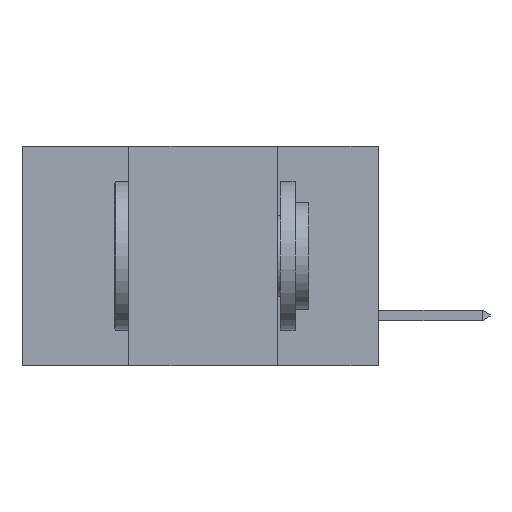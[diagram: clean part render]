
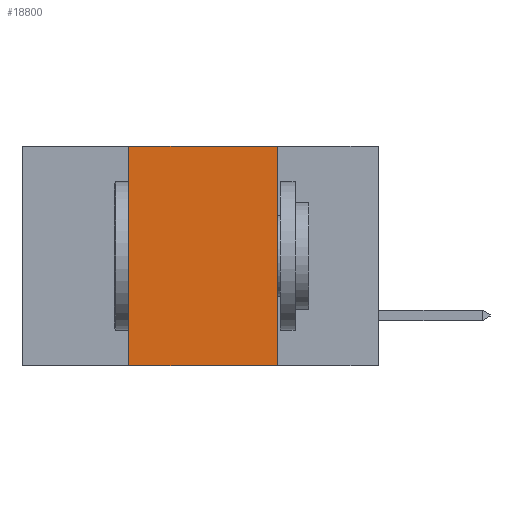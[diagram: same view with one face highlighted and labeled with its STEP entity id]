
A CAD part, left-side view. The second image highlights one B-rep face of the part: STEP entity #18800.
In plain terms, the highlighted planar face has unit normal (-1, 0, 0).
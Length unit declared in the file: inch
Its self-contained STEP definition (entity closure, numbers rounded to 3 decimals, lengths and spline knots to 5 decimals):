
#1243 = AXIS2_PLACEMENT_3D ( 'NONE', #8202, #19366, #8288 ) ;
#2293 = ORIENTED_EDGE ( 'NONE', *, *, #5641, .F. ) ;
#2319 = DIRECTION ( 'NONE',  ( 0., 0., 1. ) ) ;
#3098 = EDGE_CURVE ( 'NONE', #23307, #8638, #22812, .T. ) ;
#4354 = EDGE_CURVE ( 'NONE', #23307, #5265, #14156, .T. ) ;
#4547 = CARTESIAN_POINT ( 'NONE',  ( 0., 0.17, 0. ) ) ;
#5265 = VERTEX_POINT ( 'NONE', #8289 ) ;
#5309 = ORIENTED_EDGE ( 'NONE', *, *, #4354, .F. ) ;
#5473 = CARTESIAN_POINT ( 'NONE',  ( 0., 0.42, -0.37 ) ) ;
#5641 = EDGE_CURVE ( 'NONE', #20863, #8638, #9137, .T. ) ;
#6243 = FACE_OUTER_BOUND ( 'NONE', #12476, .T. ) ;
#6363 = PLANE ( 'NONE',  #1243 ) ;
#8202 = CARTESIAN_POINT ( 'NONE',  ( 0., 0.6, 0. ) ) ;
#8288 = DIRECTION ( 'NONE',  ( 0., 0., -1. ) ) ;
#8289 = CARTESIAN_POINT ( 'NONE',  ( 0., 0.42, 0. ) ) ;
#8351 = DIRECTION ( 'NONE',  ( 0., 0., -1. ) ) ;
#8638 = VERTEX_POINT ( 'NONE', #11165 ) ;
#9137 = LINE ( 'NONE', #4547, #23257 ) ;
#9141 = ORIENTED_EDGE ( 'NONE', *, *, #24098, .F. ) ;
#9716 = CARTESIAN_POINT ( 'NONE',  ( 0., 0.6, 0. ) ) ;
#11165 = CARTESIAN_POINT ( 'NONE',  ( 0., 0.17, -0.37 ) ) ;
#11465 = VECTOR ( 'NONE', #11610, 39.37008 ) ;
#11610 = DIRECTION ( 'NONE',  ( 0., -1., 0. ) ) ;
#11720 = CARTESIAN_POINT ( 'NONE',  ( 0., 0.6, -0.37 ) ) ;
#12476 = EDGE_LOOP ( 'NONE', ( #2293, #9141, #5309, #21863 ) ) ;
#12656 = CARTESIAN_POINT ( 'NONE',  ( 0., 0.17, 0. ) ) ;
#12867 = CARTESIAN_POINT ( 'NONE',  ( 0., 0.42, 0. ) ) ;
#13573 = VECTOR ( 'NONE', #2319, 39.37008 ) ;
#13644 = VECTOR ( 'NONE', #15431, 39.37008 ) ;
#14156 = LINE ( 'NONE', #12867, #13573 ) ;
#15431 = DIRECTION ( 'NONE',  ( 0., -1., 0. ) ) ;
#16360 = LINE ( 'NONE', #9716, #11465 ) ;
#18800 = ADVANCED_FACE ( 'NONE', ( #6243 ), #6363, .F. ) ;
#19366 = DIRECTION ( 'NONE',  ( 1., 0., 0. ) ) ;
#20863 = VERTEX_POINT ( 'NONE', #12656 ) ;
#21863 = ORIENTED_EDGE ( 'NONE', *, *, #3098, .T. ) ;
#22812 = LINE ( 'NONE', #11720, #13644 ) ;
#23257 = VECTOR ( 'NONE', #8351, 39.37008 ) ;
#23307 = VERTEX_POINT ( 'NONE', #5473 ) ;
#24098 = EDGE_CURVE ( 'NONE', #5265, #20863, #16360, .T. ) ;
